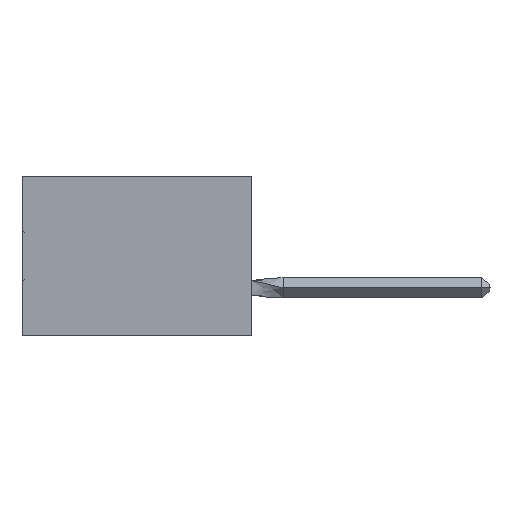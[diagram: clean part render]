
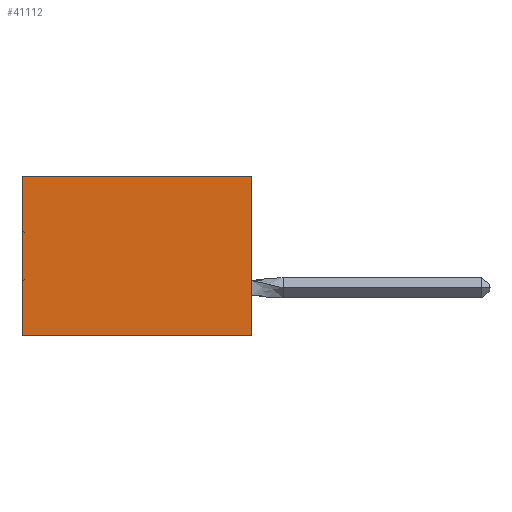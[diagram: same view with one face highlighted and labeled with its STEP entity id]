
A CAD part, left-side view. The second image highlights one B-rep face of the part: STEP entity #41112.
In plain terms, the highlighted planar face has unit normal (-1, 0, 0).
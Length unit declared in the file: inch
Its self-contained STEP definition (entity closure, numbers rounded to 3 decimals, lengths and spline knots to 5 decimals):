
#193 = ORIENTED_EDGE ( 'NONE', *, *, #29356, .T. ) ;
#1603 = LINE ( 'NONE', #11319, #44233 ) ;
#2583 = VERTEX_POINT ( 'NONE', #8011 ) ;
#5183 = CARTESIAN_POINT ( 'NONE',  ( 0.305, 0.72, 0. ) ) ;
#6527 = EDGE_CURVE ( 'NONE', #16798, #2583, #1603, .T. ) ;
#6696 = EDGE_LOOP ( 'NONE', ( #20254, #23552, #36083, #193 ) ) ;
#8011 = CARTESIAN_POINT ( 'NONE',  ( 0.305, 0.72, -0.5 ) ) ;
#9703 = AXIS2_PLACEMENT_3D ( 'NONE', #50912, #16245, #16442 ) ;
#9788 = DIRECTION ( 'NONE',  ( 0., 0., -1. ) ) ;
#11319 = CARTESIAN_POINT ( 'NONE',  ( 0.305, 0., -0.5 ) ) ;
#15413 = LINE ( 'NONE', #18104, #22786 ) ;
#15705 = EDGE_CURVE ( 'NONE', #18429, #16798, #21814, .T. ) ;
#16245 = DIRECTION ( 'NONE',  ( 1., 0., 0. ) ) ;
#16442 = DIRECTION ( 'NONE',  ( 0., 0., -1. ) ) ;
#16798 = VERTEX_POINT ( 'NONE', #19845 ) ;
#18104 = CARTESIAN_POINT ( 'NONE',  ( 0.305, 0., 0. ) ) ;
#18429 = VERTEX_POINT ( 'NONE', #28227 ) ;
#19816 = FACE_OUTER_BOUND ( 'NONE', #6696, .T. ) ;
#19845 = CARTESIAN_POINT ( 'NONE',  ( 0.305, 0., -0.5 ) ) ;
#20254 = ORIENTED_EDGE ( 'NONE', *, *, #32659, .T. ) ;
#21814 = LINE ( 'NONE', #35219, #45015 ) ;
#22786 = VECTOR ( 'NONE', #34549, 39.37008 ) ;
#23552 = ORIENTED_EDGE ( 'NONE', *, *, #6527, .F. ) ;
#28227 = CARTESIAN_POINT ( 'NONE',  ( 0.305, 0., 0. ) ) ;
#29356 = EDGE_CURVE ( 'NONE', #18429, #39974, #15413, .T. ) ;
#32659 = EDGE_CURVE ( 'NONE', #39974, #2583, #34644, .T. ) ;
#32882 = DIRECTION ( 'NONE',  ( 0., 1., 0. ) ) ;
#34549 = DIRECTION ( 'NONE',  ( 0., 1., 0. ) ) ;
#34644 = LINE ( 'NONE', #38546, #51441 ) ;
#35219 = CARTESIAN_POINT ( 'NONE',  ( 0.305, 0., -0.5 ) ) ;
#36083 = ORIENTED_EDGE ( 'NONE', *, *, #15705, .F. ) ;
#38546 = CARTESIAN_POINT ( 'NONE',  ( 0.305, 0.72, -0.5 ) ) ;
#39974 = VERTEX_POINT ( 'NONE', #5183 ) ;
#41112 = ADVANCED_FACE ( 'NONE', ( #19816 ), #45837, .F. ) ;
#44233 = VECTOR ( 'NONE', #32882, 39.37008 ) ;
#45015 = VECTOR ( 'NONE', #9788, 39.37008 ) ;
#45837 = PLANE ( 'NONE',  #9703 ) ;
#46971 = DIRECTION ( 'NONE',  ( 0., 0., -1. ) ) ;
#50912 = CARTESIAN_POINT ( 'NONE',  ( 0.305, 0., -0.5 ) ) ;
#51441 = VECTOR ( 'NONE', #46971, 39.37008 ) ;
